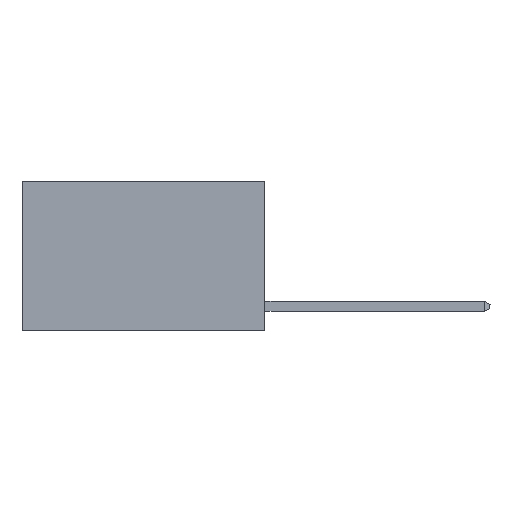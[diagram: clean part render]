
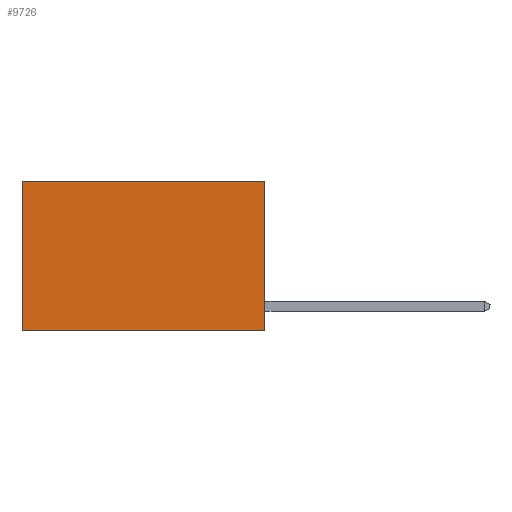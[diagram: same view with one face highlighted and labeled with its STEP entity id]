
A CAD part, left-side view. The second image highlights one B-rep face of the part: STEP entity #9726.
In plain terms, the highlighted planar face has unit normal (-1, 0, 0).
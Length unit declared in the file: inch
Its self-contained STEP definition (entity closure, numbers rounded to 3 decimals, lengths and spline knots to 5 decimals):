
#782 = CARTESIAN_POINT ( 'NONE',  ( 0.2625, 0., 0. ) ) ;
#909 = ORIENTED_EDGE ( 'NONE', *, *, #27185, .F. ) ;
#1894 = ORIENTED_EDGE ( 'NONE', *, *, #10396, .T. ) ;
#2781 = DIRECTION ( 'NONE',  ( 0., 0., -1. ) ) ;
#3012 = LINE ( 'NONE', #782, #5330 ) ;
#3646 = CARTESIAN_POINT ( 'NONE',  ( 0.2625, 0., 0. ) ) ;
#5060 = VECTOR ( 'NONE', #11446, 39.37008 ) ;
#5330 = VECTOR ( 'NONE', #14476, 39.37008 ) ;
#6616 = LINE ( 'NONE', #28659, #11331 ) ;
#6928 = VERTEX_POINT ( 'NONE', #20067 ) ;
#6932 = CARTESIAN_POINT ( 'NONE',  ( 0.2625, 0., -0.37 ) ) ;
#7300 = VERTEX_POINT ( 'NONE', #13096 ) ;
#9726 = ADVANCED_FACE ( 'NONE', ( #12663 ), #21481, .F. ) ;
#10396 = EDGE_CURVE ( 'NONE', #6928, #23320, #20571, .T. ) ;
#11331 = VECTOR ( 'NONE', #2781, 39.37008 ) ;
#11446 = DIRECTION ( 'NONE',  ( 0., 0., -1. ) ) ;
#12663 = FACE_OUTER_BOUND ( 'NONE', #24003, .T. ) ;
#13096 = CARTESIAN_POINT ( 'NONE',  ( 0.2625, 0., -0.37 ) ) ;
#13461 = LINE ( 'NONE', #6932, #22212 ) ;
#13709 = EDGE_CURVE ( 'NONE', #15424, #6928, #3012, .T. ) ;
#14476 = DIRECTION ( 'NONE',  ( 0., 1., 0. ) ) ;
#15424 = VERTEX_POINT ( 'NONE', #15705 ) ;
#15705 = CARTESIAN_POINT ( 'NONE',  ( 0.2625, 0., 0. ) ) ;
#15811 = CARTESIAN_POINT ( 'NONE',  ( 0.2625, 0.6, 0. ) ) ;
#15830 = ORIENTED_EDGE ( 'NONE', *, *, #13709, .T. ) ;
#16050 = DIRECTION ( 'NONE',  ( 0., 1., 0. ) ) ;
#18508 = CARTESIAN_POINT ( 'NONE',  ( 0.2625, 0.6, -0.37 ) ) ;
#19317 = DIRECTION ( 'NONE',  ( 0., 0., -1. ) ) ;
#20067 = CARTESIAN_POINT ( 'NONE',  ( 0.2625, 0.6, 0. ) ) ;
#20571 = LINE ( 'NONE', #15811, #5060 ) ;
#20721 = EDGE_CURVE ( 'NONE', #15424, #7300, #6616, .T. ) ;
#21481 = PLANE ( 'NONE',  #28672 ) ;
#22212 = VECTOR ( 'NONE', #16050, 39.37008 ) ;
#23320 = VERTEX_POINT ( 'NONE', #18508 ) ;
#23523 = DIRECTION ( 'NONE',  ( 1., 0., 0. ) ) ;
#24003 = EDGE_LOOP ( 'NONE', ( #1894, #909, #28623, #15830 ) ) ;
#27185 = EDGE_CURVE ( 'NONE', #7300, #23320, #13461, .T. ) ;
#28623 = ORIENTED_EDGE ( 'NONE', *, *, #20721, .F. ) ;
#28659 = CARTESIAN_POINT ( 'NONE',  ( 0.2625, 0., 0. ) ) ;
#28672 = AXIS2_PLACEMENT_3D ( 'NONE', #3646, #23523, #19317 ) ;
